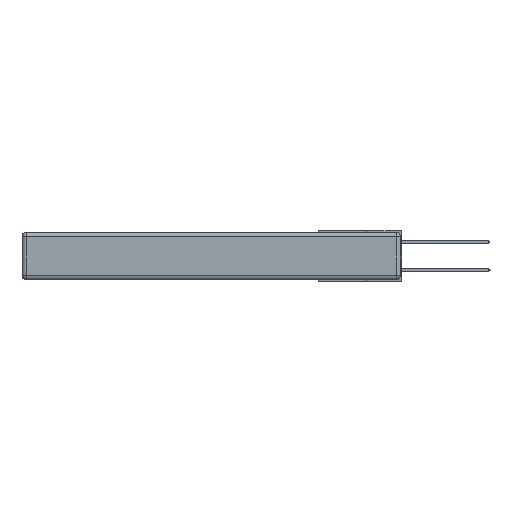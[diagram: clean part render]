
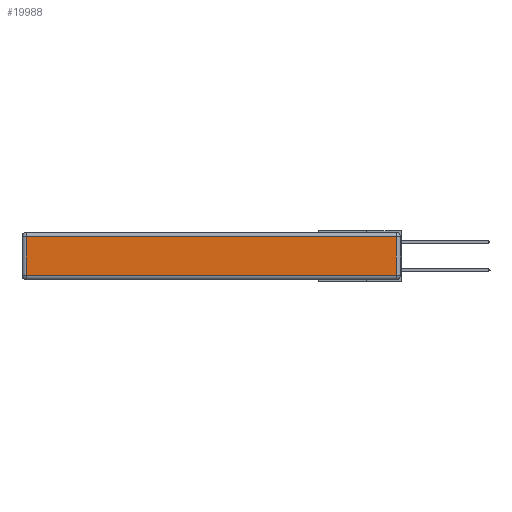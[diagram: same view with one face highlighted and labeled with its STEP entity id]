
A CAD part, left-side view. The second image highlights one B-rep face of the part: STEP entity #19988.
In plain terms, the highlighted planar face has unit normal (-1, 0, 0).
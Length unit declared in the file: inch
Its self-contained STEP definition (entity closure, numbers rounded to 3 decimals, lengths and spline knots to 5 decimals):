
#162 = DIRECTION ( 'NONE',  ( -1., 0., 0. ) ) ;
#164 = CARTESIAN_POINT ( 'NONE',  ( 0., 0.03, -0.03 ) ) ;
#447 = VERTEX_POINT ( 'NONE', #164 ) ;
#1509 = CARTESIAN_POINT ( 'NONE',  ( 0., 2.72, -0.03 ) ) ;
#1989 = CARTESIAN_POINT ( 'NONE',  ( 0., 2.72, -0.313 ) ) ;
#3138 = LINE ( 'NONE', #11103, #15491 ) ;
#4024 = VERTEX_POINT ( 'NONE', #10498 ) ;
#4146 = DIRECTION ( 'NONE',  ( 0., 0., -1. ) ) ;
#4636 = ORIENTED_EDGE ( 'NONE', *, *, #11385, .T. ) ;
#4825 = PLANE ( 'NONE',  #9917 ) ;
#4896 = CARTESIAN_POINT ( 'NONE',  ( 0., 0., -0.343 ) ) ;
#6096 = LINE ( 'NONE', #13589, #8808 ) ;
#8146 = DIRECTION ( 'NONE',  ( 0., 0., 1. ) ) ;
#8319 = LINE ( 'NONE', #13313, #8801 ) ;
#8353 = ORIENTED_EDGE ( 'NONE', *, *, #12614, .T. ) ;
#8537 = EDGE_CURVE ( 'NONE', #447, #9393, #6096, .T. ) ;
#8602 = ORIENTED_EDGE ( 'NONE', *, *, #10876, .T. ) ;
#8801 = VECTOR ( 'NONE', #18152, 39.37008 ) ;
#8808 = VECTOR ( 'NONE', #10300, 39.37008 ) ;
#9393 = VERTEX_POINT ( 'NONE', #1509 ) ;
#9572 = VERTEX_POINT ( 'NONE', #1989 ) ;
#9917 = AXIS2_PLACEMENT_3D ( 'NONE', #4896, #162, #8146 ) ;
#9989 = LINE ( 'NONE', #10516, #16152 ) ;
#10300 = DIRECTION ( 'NONE',  ( 0., 1., 0. ) ) ;
#10498 = CARTESIAN_POINT ( 'NONE',  ( 0., 0.03, -0.313 ) ) ;
#10516 = CARTESIAN_POINT ( 'NONE',  ( 0., 2.72, -0.343 ) ) ;
#10876 = EDGE_CURVE ( 'NONE', #4024, #447, #3138, .T. ) ;
#11103 = CARTESIAN_POINT ( 'NONE',  ( 0., 0.03, -0.343 ) ) ;
#11385 = EDGE_CURVE ( 'NONE', #9572, #4024, #8319, .T. ) ;
#12614 = EDGE_CURVE ( 'NONE', #9393, #9572, #9989, .T. ) ;
#12651 = DIRECTION ( 'NONE',  ( 0., 0., 1. ) ) ;
#13313 = CARTESIAN_POINT ( 'NONE',  ( 0., 0., -0.313 ) ) ;
#13589 = CARTESIAN_POINT ( 'NONE',  ( 0., 2.75, -0.03 ) ) ;
#15491 = VECTOR ( 'NONE', #12651, 39.37008 ) ;
#15535 = FACE_OUTER_BOUND ( 'NONE', #15954, .T. ) ;
#15954 = EDGE_LOOP ( 'NONE', ( #4636, #8602, #18534, #8353 ) ) ;
#16152 = VECTOR ( 'NONE', #4146, 39.37008 ) ;
#18152 = DIRECTION ( 'NONE',  ( 0., -1., 0. ) ) ;
#18534 = ORIENTED_EDGE ( 'NONE', *, *, #8537, .T. ) ;
#19988 = ADVANCED_FACE ( 'NONE', ( #15535 ), #4825, .T. ) ;
